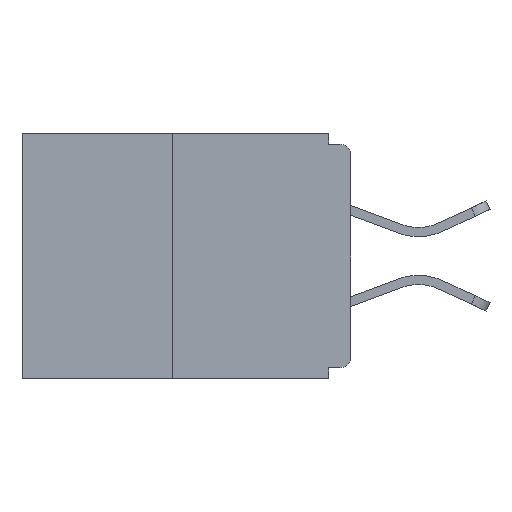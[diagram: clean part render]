
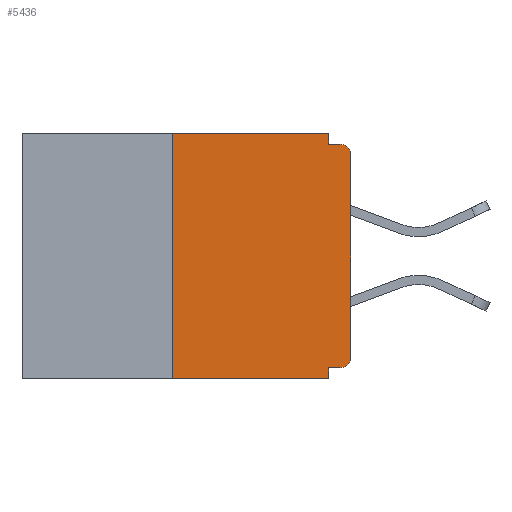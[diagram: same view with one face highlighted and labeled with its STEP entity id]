
A CAD part, left-side view. The second image highlights one B-rep face of the part: STEP entity #5436.
In plain terms, the highlighted planar face has unit normal (-1, 0, 0).
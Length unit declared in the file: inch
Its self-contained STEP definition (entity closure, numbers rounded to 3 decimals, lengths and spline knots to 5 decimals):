
#636 = EDGE_CURVE ( 'NONE', #9962, #6663, #9511, .T. ) ;
#653 = EDGE_CURVE ( 'NONE', #8489, #8978, #7599, .T. ) ;
#670 = VERTEX_POINT ( 'NONE', #11056 ) ;
#700 = VERTEX_POINT ( 'NONE', #3658 ) ;
#748 = CARTESIAN_POINT ( 'NONE',  ( 0., 0.031, -0.328 ) ) ;
#866 = ORIENTED_EDGE ( 'NONE', *, *, #12000, .T. ) ;
#1087 = DIRECTION ( 'NONE',  ( 0., -1., 0. ) ) ;
#1386 = AXIS2_PLACEMENT_3D ( 'NONE', #7482, #10310, #7406 ) ;
#1448 = DIRECTION ( 'NONE',  ( 0., 0., 1. ) ) ;
#1648 = EDGE_CURVE ( 'NONE', #670, #700, #6636, .T. ) ;
#1663 = CARTESIAN_POINT ( 'NONE',  ( 0., 0.46, 0. ) ) ;
#1886 = CARTESIAN_POINT ( 'NONE',  ( 0., 0.015, -0.313 ) ) ;
#2306 = VECTOR ( 'NONE', #9402, 39.37008 ) ;
#2328 = VECTOR ( 'NONE', #10790, 39.37008 ) ;
#2661 = AXIS2_PLACEMENT_3D ( 'NONE', #8469, #5742, #2928 ) ;
#2826 = DIRECTION ( 'NONE',  ( -1., 0., 0. ) ) ;
#2928 = DIRECTION ( 'NONE',  ( 0., 0., -1. ) ) ;
#2966 = CARTESIAN_POINT ( 'NONE',  ( 0., 0.25, 0. ) ) ;
#3333 = CARTESIAN_POINT ( 'NONE',  ( 0., 0., -0.313 ) ) ;
#3503 = CARTESIAN_POINT ( 'NONE',  ( 0., 0.031, -0.343 ) ) ;
#3541 = VECTOR ( 'NONE', #10937, 39.37008 ) ;
#3579 = EDGE_CURVE ( 'NONE', #9733, #9962, #11269, .T. ) ;
#3585 = EDGE_LOOP ( 'NONE', ( #5357, #7374, #866, #9028, #9471, #4735, #5383, #10003, #4461, #7782 ) ) ;
#3658 = CARTESIAN_POINT ( 'NONE',  ( 0., 0.015, -0.015 ) ) ;
#3782 = CARTESIAN_POINT ( 'NONE',  ( 0., 0., -0.015 ) ) ;
#4001 = AXIS2_PLACEMENT_3D ( 'NONE', #1886, #2826, #9329 ) ;
#4461 = ORIENTED_EDGE ( 'NONE', *, *, #1648, .F. ) ;
#4505 = DIRECTION ( 'NONE',  ( 0., 0., -1. ) ) ;
#4735 = ORIENTED_EDGE ( 'NONE', *, *, #10839, .T. ) ;
#4781 = CIRCLE ( 'NONE', #4001, 0.015 ) ;
#4973 = DIRECTION ( 'NONE',  ( 0., 1., 0. ) ) ;
#5037 = VERTEX_POINT ( 'NONE', #11613 ) ;
#5041 = CARTESIAN_POINT ( 'NONE',  ( 0., 0.031, 0. ) ) ;
#5085 = FACE_OUTER_BOUND ( 'NONE', #3585, .T. ) ;
#5213 = EDGE_CURVE ( 'NONE', #7820, #8489, #5229, .T. ) ;
#5229 = LINE ( 'NONE', #8950, #11371 ) ;
#5285 = VECTOR ( 'NONE', #4973, 39.37008 ) ;
#5357 = ORIENTED_EDGE ( 'NONE', *, *, #653, .F. ) ;
#5383 = ORIENTED_EDGE ( 'NONE', *, *, #10550, .T. ) ;
#5436 = ADVANCED_FACE ( 'NONE', ( #5085 ), #7361, .F. ) ;
#5461 = CARTESIAN_POINT ( 'NONE',  ( 0., 0.25, -0.343 ) ) ;
#5742 = DIRECTION ( 'NONE',  ( -1., 0., 0. ) ) ;
#6052 = LINE ( 'NONE', #8127, #2306 ) ;
#6352 = VECTOR ( 'NONE', #11327, 39.37008 ) ;
#6636 = LINE ( 'NONE', #3782, #7936 ) ;
#6663 = VERTEX_POINT ( 'NONE', #10285 ) ;
#7292 = VECTOR ( 'NONE', #4505, 39.37008 ) ;
#7361 = PLANE ( 'NONE',  #1386 ) ;
#7374 = ORIENTED_EDGE ( 'NONE', *, *, #5213, .F. ) ;
#7406 = DIRECTION ( 'NONE',  ( 0., 0., -1. ) ) ;
#7482 = CARTESIAN_POINT ( 'NONE',  ( 0., 0.46, 0. ) ) ;
#7599 = LINE ( 'NONE', #1663, #3541 ) ;
#7733 = CARTESIAN_POINT ( 'NONE',  ( 0., 0., -0.328 ) ) ;
#7782 = ORIENTED_EDGE ( 'NONE', *, *, #7885, .F. ) ;
#7820 = VERTEX_POINT ( 'NONE', #5461 ) ;
#7885 = EDGE_CURVE ( 'NONE', #8978, #670, #11335, .T. ) ;
#7936 = VECTOR ( 'NONE', #1087, 39.37008 ) ;
#8127 = CARTESIAN_POINT ( 'NONE',  ( 0., 0.46, -0.343 ) ) ;
#8469 = CARTESIAN_POINT ( 'NONE',  ( 0., 0.015, -0.03 ) ) ;
#8489 = VERTEX_POINT ( 'NONE', #2966 ) ;
#8514 = CARTESIAN_POINT ( 'NONE',  ( 0., 0.015, -0.328 ) ) ;
#8950 = CARTESIAN_POINT ( 'NONE',  ( 0., 0.25, 0. ) ) ;
#8978 = VERTEX_POINT ( 'NONE', #10186 ) ;
#9028 = ORIENTED_EDGE ( 'NONE', *, *, #636, .F. ) ;
#9329 = DIRECTION ( 'NONE',  ( 0., 0., -1. ) ) ;
#9402 = DIRECTION ( 'NONE',  ( 0., -1., 0. ) ) ;
#9471 = ORIENTED_EDGE ( 'NONE', *, *, #3579, .F. ) ;
#9511 = LINE ( 'NONE', #3503, #7292 ) ;
#9733 = VERTEX_POINT ( 'NONE', #8514 ) ;
#9755 = LINE ( 'NONE', #9865, #2328 ) ;
#9865 = CARTESIAN_POINT ( 'NONE',  ( 0., 0., 0. ) ) ;
#9962 = VERTEX_POINT ( 'NONE', #748 ) ;
#10003 = ORIENTED_EDGE ( 'NONE', *, *, #10180, .T. ) ;
#10180 = EDGE_CURVE ( 'NONE', #5037, #700, #11649, .T. ) ;
#10186 = CARTESIAN_POINT ( 'NONE',  ( 0., 0.031, 0. ) ) ;
#10285 = CARTESIAN_POINT ( 'NONE',  ( 0., 0.031, -0.343 ) ) ;
#10310 = DIRECTION ( 'NONE',  ( 1., 0., 0. ) ) ;
#10550 = EDGE_CURVE ( 'NONE', #11144, #5037, #9755, .T. ) ;
#10790 = DIRECTION ( 'NONE',  ( 0., 0., 1. ) ) ;
#10839 = EDGE_CURVE ( 'NONE', #9733, #11144, #4781, .T. ) ;
#10937 = DIRECTION ( 'NONE',  ( 0., -1., 0. ) ) ;
#11056 = CARTESIAN_POINT ( 'NONE',  ( 0., 0.031, -0.015 ) ) ;
#11144 = VERTEX_POINT ( 'NONE', #3333 ) ;
#11269 = LINE ( 'NONE', #7733, #5285 ) ;
#11327 = DIRECTION ( 'NONE',  ( 0., 0., -1. ) ) ;
#11335 = LINE ( 'NONE', #5041, #6352 ) ;
#11371 = VECTOR ( 'NONE', #1448, 39.37008 ) ;
#11613 = CARTESIAN_POINT ( 'NONE',  ( 0., 0., -0.03 ) ) ;
#11649 = CIRCLE ( 'NONE', #2661, 0.015 ) ;
#12000 = EDGE_CURVE ( 'NONE', #7820, #6663, #6052, .T. ) ;
